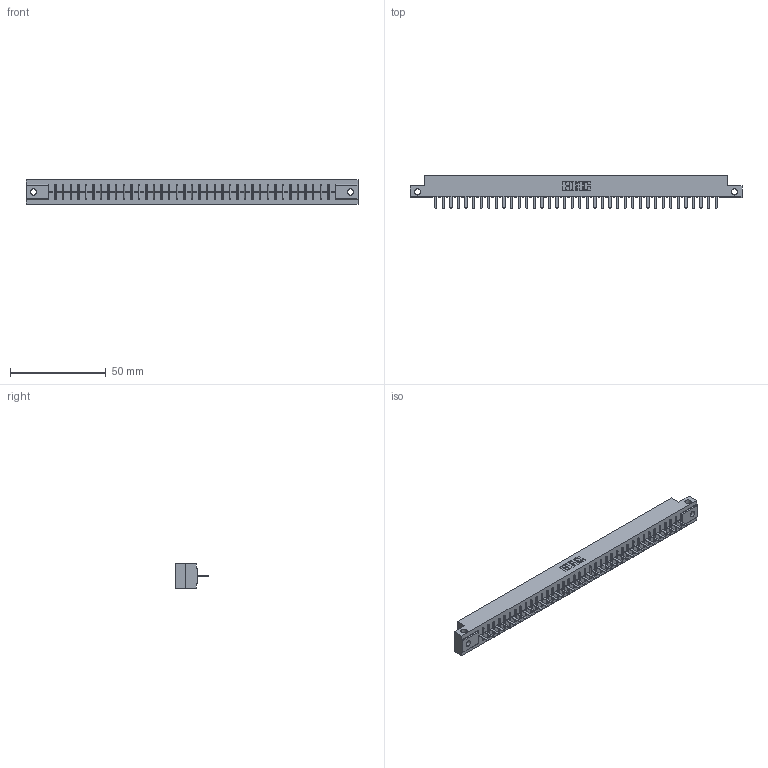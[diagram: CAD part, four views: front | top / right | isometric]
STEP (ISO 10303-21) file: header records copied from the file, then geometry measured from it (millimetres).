
FILE_DESCRIPTION (( 'STEP AP203' ), '1' );
FILE_NAME ('306-038-420-112.STEP', '2020-09-22T05:37:54', ( '' ), ( '' ), 'SwSTEP 2.0', 'SolidWorks 2020', '' );
FILE_SCHEMA (( 'CONFIG_CONTROL_DESIGN' ));
Length unit declared in the file: inch
Products named in the file (3): 306 Part_.128 Dia; 306-290-001_120; 306-038-420-112
Assembly tree (39 placements, depth 2):
  306-038-420-112
    306 Part_.128 Dia
    306-290-001_120  x38
Bounding box: 173.58 x 17.12 x 12.7 mm (x, y, z)
Volume: 18962.9 mm3; surface area: 19474.2 mm2
Topology: 39 solids, 39 shells, 2788 faces, 7838 edges, 5016 vertices
Faces by surface type: plane 1854, cylinder 782, sphere 152
Entity records: 36317 total; most frequent: CARTESIAN_POINT 6145, ORIENTED_EDGE 6048, DIRECTION 5998, EDGE_CURVE 3024, LINE 2348, VECTOR 2348, VERTEX_POINT 1908, AXIS2_PLACEMENT_3D 1825
